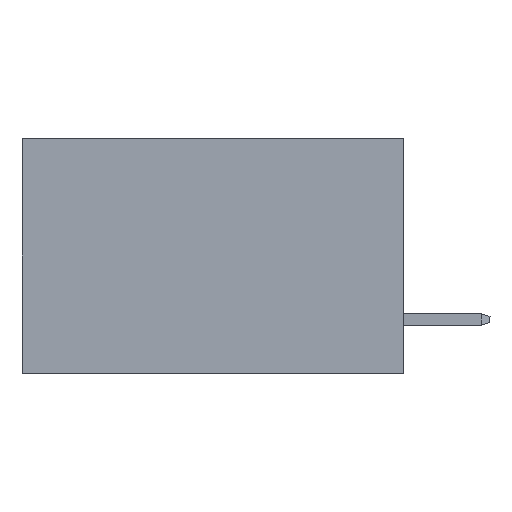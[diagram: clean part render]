
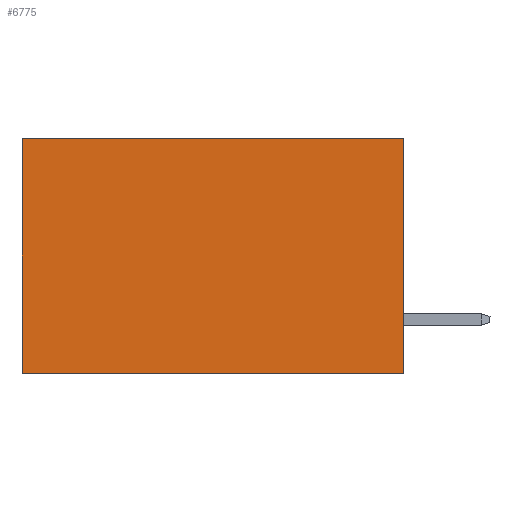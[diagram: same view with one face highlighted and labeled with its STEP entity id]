
A CAD part, left-side view. The second image highlights one B-rep face of the part: STEP entity #6775.
In plain terms, the highlighted planar face has unit normal (-1, 0, 0).
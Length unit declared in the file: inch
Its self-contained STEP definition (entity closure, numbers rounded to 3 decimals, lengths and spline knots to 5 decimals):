
#215 = CARTESIAN_POINT ( 'NONE',  ( 0.2875, 0., 0. ) ) ;
#834 = DIRECTION ( 'NONE',  ( 1., 0., 0. ) ) ;
#1230 = DIRECTION ( 'NONE',  ( 0., 0., -1. ) ) ;
#1618 = VECTOR ( 'NONE', #5483, 39.37008 ) ;
#1810 = VECTOR ( 'NONE', #11861, 39.37008 ) ;
#1917 = EDGE_CURVE ( 'NONE', #11624, #2497, #7118, .T. ) ;
#2497 = VERTEX_POINT ( 'NONE', #9242 ) ;
#3001 = DIRECTION ( 'NONE',  ( 0., 0., -1. ) ) ;
#3629 = EDGE_CURVE ( 'NONE', #2497, #10220, #4240, .T. ) ;
#4176 = EDGE_CURVE ( 'NONE', #11624, #7835, #11339, .T. ) ;
#4240 = LINE ( 'NONE', #11272, #4781 ) ;
#4767 = PLANE ( 'NONE',  #5326 ) ;
#4781 = VECTOR ( 'NONE', #1230, 39.37008 ) ;
#4877 = ORIENTED_EDGE ( 'NONE', *, *, #3629, .T. ) ;
#5326 = AXIS2_PLACEMENT_3D ( 'NONE', #9897, #834, #3001 ) ;
#5483 = DIRECTION ( 'NONE',  ( 0., 0., -1. ) ) ;
#5669 = ORIENTED_EDGE ( 'NONE', *, *, #7297, .F. ) ;
#5965 = ORIENTED_EDGE ( 'NONE', *, *, #1917, .T. ) ;
#6162 = CARTESIAN_POINT ( 'NONE',  ( 0.2875, 0., -0.37 ) ) ;
#6181 = LINE ( 'NONE', #12042, #12819 ) ;
#6775 = ADVANCED_FACE ( 'NONE', ( #12642 ), #4767, .F. ) ;
#6983 = EDGE_LOOP ( 'NONE', ( #4877, #5669, #10698, #5965 ) ) ;
#7118 = LINE ( 'NONE', #215, #1810 ) ;
#7297 = EDGE_CURVE ( 'NONE', #7835, #10220, #6181, .T. ) ;
#7835 = VERTEX_POINT ( 'NONE', #6162 ) ;
#9045 = DIRECTION ( 'NONE',  ( 0., 1., 0. ) ) ;
#9242 = CARTESIAN_POINT ( 'NONE',  ( 0.2875, 0.6, 0. ) ) ;
#9484 = CARTESIAN_POINT ( 'NONE',  ( 0.2875, 0.6, -0.37 ) ) ;
#9897 = CARTESIAN_POINT ( 'NONE',  ( 0.2875, 0., 0. ) ) ;
#10220 = VERTEX_POINT ( 'NONE', #9484 ) ;
#10698 = ORIENTED_EDGE ( 'NONE', *, *, #4176, .F. ) ;
#10859 = CARTESIAN_POINT ( 'NONE',  ( 0.2875, 0., 0. ) ) ;
#11272 = CARTESIAN_POINT ( 'NONE',  ( 0.2875, 0.6, 0. ) ) ;
#11339 = LINE ( 'NONE', #11473, #1618 ) ;
#11473 = CARTESIAN_POINT ( 'NONE',  ( 0.2875, 0., 0. ) ) ;
#11624 = VERTEX_POINT ( 'NONE', #10859 ) ;
#11861 = DIRECTION ( 'NONE',  ( 0., 1., 0. ) ) ;
#12042 = CARTESIAN_POINT ( 'NONE',  ( 0.2875, 0., -0.37 ) ) ;
#12642 = FACE_OUTER_BOUND ( 'NONE', #6983, .T. ) ;
#12819 = VECTOR ( 'NONE', #9045, 39.37008 ) ;
